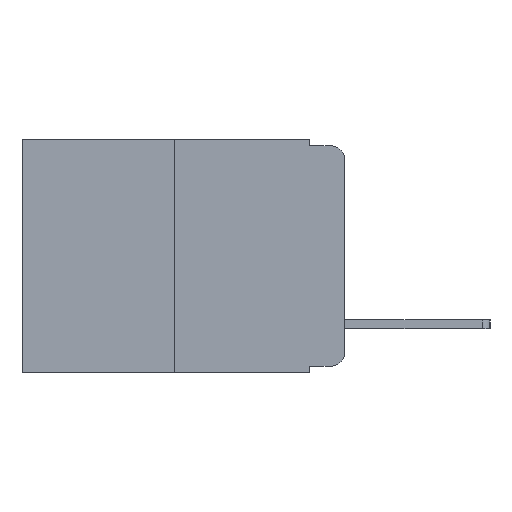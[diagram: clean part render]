
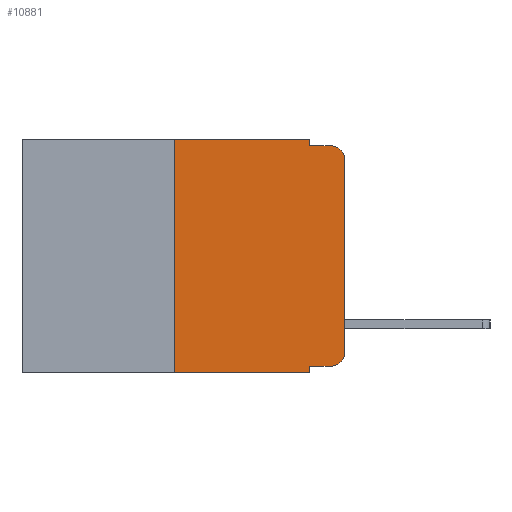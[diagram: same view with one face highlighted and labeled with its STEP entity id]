
A CAD part, left-side view. The second image highlights one B-rep face of the part: STEP entity #10881.
In plain terms, the highlighted planar face has unit normal (-1, 0, 0).
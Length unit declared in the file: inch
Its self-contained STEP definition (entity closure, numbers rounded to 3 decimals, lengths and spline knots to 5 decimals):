
#519 = CARTESIAN_POINT ( 'NONE',  ( 0., 0.051, 0. ) ) ;
#720 = CARTESIAN_POINT ( 'NONE',  ( 0., 0.473, 0. ) ) ;
#966 = DIRECTION ( 'NONE',  ( -1., 0., 0. ) ) ;
#1611 = ORIENTED_EDGE ( 'NONE', *, *, #24712, .T. ) ;
#1722 = CARTESIAN_POINT ( 'NONE',  ( 0., 0.051, -0.333 ) ) ;
#2758 = DIRECTION ( 'NONE',  ( 0., 0., -1. ) ) ;
#3170 = VERTEX_POINT ( 'NONE', #5071 ) ;
#3267 = EDGE_CURVE ( 'NONE', #7849, #6151, #15096, .T. ) ;
#3387 = DIRECTION ( 'NONE',  ( 0., 0., 1. ) ) ;
#3819 = VERTEX_POINT ( 'NONE', #519 ) ;
#4740 = EDGE_CURVE ( 'NONE', #6037, #11608, #12651, .T. ) ;
#5071 = CARTESIAN_POINT ( 'NONE',  ( 0., 0.02, -0.333 ) ) ;
#5111 = DIRECTION ( 'NONE',  ( 0., 0., -1. ) ) ;
#5440 = CARTESIAN_POINT ( 'NONE',  ( 0., 0.02, -0.03 ) ) ;
#5723 = CARTESIAN_POINT ( 'NONE',  ( 0., 0.25, -0.343 ) ) ;
#5829 = CARTESIAN_POINT ( 'NONE',  ( 0., 0.25, 0. ) ) ;
#6037 = VERTEX_POINT ( 'NONE', #19719 ) ;
#6151 = VERTEX_POINT ( 'NONE', #23759 ) ;
#6322 = ORIENTED_EDGE ( 'NONE', *, *, #22326, .F. ) ;
#6503 = VECTOR ( 'NONE', #17747, 39.37008 ) ;
#6888 = VECTOR ( 'NONE', #11151, 39.37008 ) ;
#6902 = VERTEX_POINT ( 'NONE', #1722 ) ;
#7279 = FACE_OUTER_BOUND ( 'NONE', #16457, .T. ) ;
#7292 = CARTESIAN_POINT ( 'NONE',  ( 0., 0.02, -0.01 ) ) ;
#7405 = DIRECTION ( 'NONE',  ( 0., 0., -1. ) ) ;
#7529 = ORIENTED_EDGE ( 'NONE', *, *, #23765, .F. ) ;
#7849 = VERTEX_POINT ( 'NONE', #5723 ) ;
#8434 = CIRCLE ( 'NONE', #19069, 0.02 ) ;
#8962 = VERTEX_POINT ( 'NONE', #11208 ) ;
#10205 = DIRECTION ( 'NONE',  ( 0., -1., 0. ) ) ;
#10706 = VECTOR ( 'NONE', #14350, 39.37008 ) ;
#10881 = ADVANCED_FACE ( 'NONE', ( #7279 ), #12527, .F. ) ;
#10895 = CARTESIAN_POINT ( 'NONE',  ( 0., 0.051, -0.343 ) ) ;
#11151 = DIRECTION ( 'NONE',  ( 0., -1., 0. ) ) ;
#11208 = CARTESIAN_POINT ( 'NONE',  ( 0., 0., -0.313 ) ) ;
#11574 = VECTOR ( 'NONE', #20394, 39.37008 ) ;
#11608 = VERTEX_POINT ( 'NONE', #7292 ) ;
#11652 = LINE ( 'NONE', #14043, #16104 ) ;
#12480 = DIRECTION ( 'NONE',  ( 0., -1., 0. ) ) ;
#12527 = PLANE ( 'NONE',  #16690 ) ;
#12651 = LINE ( 'NONE', #13087, #6888 ) ;
#12760 = CARTESIAN_POINT ( 'NONE',  ( 0., 0.02, -0.313 ) ) ;
#13087 = CARTESIAN_POINT ( 'NONE',  ( 0., 0.051, -0.01 ) ) ;
#13572 = ORIENTED_EDGE ( 'NONE', *, *, #4740, .F. ) ;
#14043 = CARTESIAN_POINT ( 'NONE',  ( 0., 0.051, -0.333 ) ) ;
#14350 = DIRECTION ( 'NONE',  ( 0., -1., 0. ) ) ;
#14429 = DIRECTION ( 'NONE',  ( 1., 0., 0. ) ) ;
#14669 = DIRECTION ( 'NONE',  ( 0., 0., -1. ) ) ;
#14686 = CIRCLE ( 'NONE', #19063, 0.02 ) ;
#14858 = CARTESIAN_POINT ( 'NONE',  ( 0., 0.051, 0. ) ) ;
#15096 = LINE ( 'NONE', #5829, #23714 ) ;
#15241 = LINE ( 'NONE', #23557, #24400 ) ;
#15670 = ORIENTED_EDGE ( 'NONE', *, *, #21308, .T. ) ;
#16104 = VECTOR ( 'NONE', #10205, 39.37008 ) ;
#16278 = EDGE_CURVE ( 'NONE', #3170, #8962, #8434, .T. ) ;
#16457 = EDGE_LOOP ( 'NONE', ( #22227, #19110, #13572, #24522, #6322, #21957, #1611, #7529, #15670, #21096 ) ) ;
#16690 = AXIS2_PLACEMENT_3D ( 'NONE', #720, #14429, #2758 ) ;
#17272 = LINE ( 'NONE', #21298, #6503 ) ;
#17629 = LINE ( 'NONE', #14858, #22450 ) ;
#17747 = DIRECTION ( 'NONE',  ( 0., 0., 1. ) ) ;
#18025 = CARTESIAN_POINT ( 'NONE',  ( 0., 0., -0.03 ) ) ;
#18069 = VERTEX_POINT ( 'NONE', #18025 ) ;
#18592 = CARTESIAN_POINT ( 'NONE',  ( 0., 0.051, 0. ) ) ;
#18809 = DIRECTION ( 'NONE',  ( -1., 0., 0. ) ) ;
#19063 = AXIS2_PLACEMENT_3D ( 'NONE', #5440, #18809, #7405 ) ;
#19069 = AXIS2_PLACEMENT_3D ( 'NONE', #12760, #966, #14669 ) ;
#19110 = ORIENTED_EDGE ( 'NONE', *, *, #20393, .T. ) ;
#19719 = CARTESIAN_POINT ( 'NONE',  ( 0., 0.051, -0.01 ) ) ;
#20393 = EDGE_CURVE ( 'NONE', #18069, #11608, #14686, .T. ) ;
#20394 = DIRECTION ( 'NONE',  ( 0., 0., -1. ) ) ;
#20626 = LINE ( 'NONE', #21673, #10706 ) ;
#20893 = LINE ( 'NONE', #18592, #11574 ) ;
#20907 = VERTEX_POINT ( 'NONE', #10895 ) ;
#21096 = ORIENTED_EDGE ( 'NONE', *, *, #16278, .T. ) ;
#21279 = EDGE_CURVE ( 'NONE', #8962, #18069, #17272, .T. ) ;
#21298 = CARTESIAN_POINT ( 'NONE',  ( 0., 0., 0. ) ) ;
#21308 = EDGE_CURVE ( 'NONE', #6902, #3170, #11652, .T. ) ;
#21673 = CARTESIAN_POINT ( 'NONE',  ( 0., 0.473, 0. ) ) ;
#21957 = ORIENTED_EDGE ( 'NONE', *, *, #3267, .F. ) ;
#22227 = ORIENTED_EDGE ( 'NONE', *, *, #21279, .T. ) ;
#22326 = EDGE_CURVE ( 'NONE', #6151, #3819, #20626, .T. ) ;
#22450 = VECTOR ( 'NONE', #5111, 39.37008 ) ;
#22538 = EDGE_CURVE ( 'NONE', #3819, #6037, #20893, .T. ) ;
#23557 = CARTESIAN_POINT ( 'NONE',  ( 0., 0.473, -0.343 ) ) ;
#23714 = VECTOR ( 'NONE', #3387, 39.37008 ) ;
#23759 = CARTESIAN_POINT ( 'NONE',  ( 0., 0.25, 0. ) ) ;
#23765 = EDGE_CURVE ( 'NONE', #6902, #20907, #17629, .T. ) ;
#24400 = VECTOR ( 'NONE', #12480, 39.37008 ) ;
#24522 = ORIENTED_EDGE ( 'NONE', *, *, #22538, .F. ) ;
#24712 = EDGE_CURVE ( 'NONE', #7849, #20907, #15241, .T. ) ;
